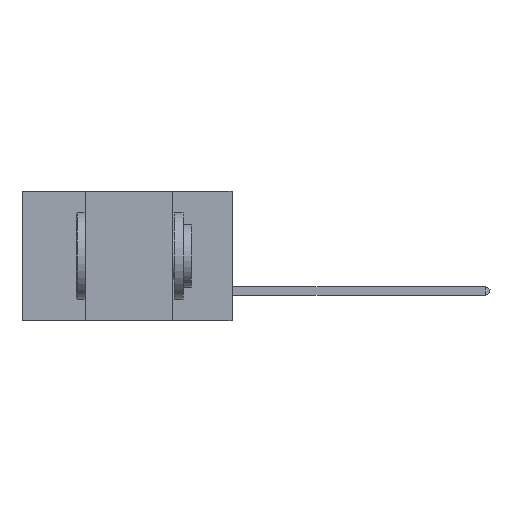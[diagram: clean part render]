
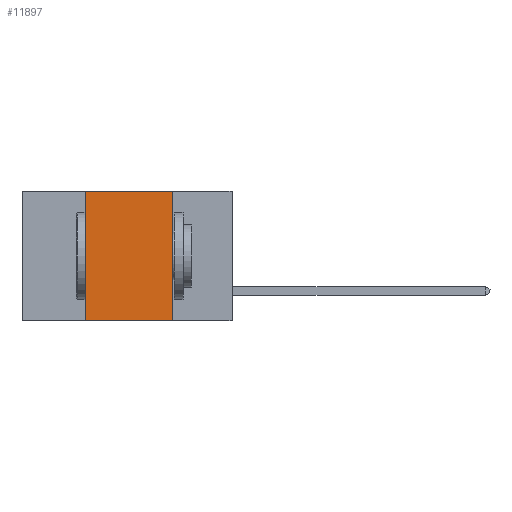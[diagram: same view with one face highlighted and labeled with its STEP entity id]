
A CAD part, left-side view. The second image highlights one B-rep face of the part: STEP entity #11897.
In plain terms, the highlighted planar face has unit normal (-1, 0, 0).
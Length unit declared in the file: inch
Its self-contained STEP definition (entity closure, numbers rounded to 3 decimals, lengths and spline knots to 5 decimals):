
#85 = DIRECTION ( 'NONE',  ( 0., 0., -1. ) ) ;
#560 = LINE ( 'NONE', #10812, #12597 ) ;
#1978 = EDGE_CURVE ( 'NONE', #9811, #10006, #11611, .T. ) ;
#2865 = DIRECTION ( 'NONE',  ( 0., 0., -1. ) ) ;
#2898 = ORIENTED_EDGE ( 'NONE', *, *, #3140, .F. ) ;
#3039 = EDGE_CURVE ( 'NONE', #12158, #3746, #560, .T. ) ;
#3117 = ORIENTED_EDGE ( 'NONE', *, *, #1978, .F. ) ;
#3140 = EDGE_CURVE ( 'NONE', #12158, #9811, #3881, .T. ) ;
#3216 = CARTESIAN_POINT ( 'NONE',  ( 0., 0.6, 0. ) ) ;
#3274 = CARTESIAN_POINT ( 'NONE',  ( 0., 0.17, 0. ) ) ;
#3532 = VECTOR ( 'NONE', #6941, 39.37008 ) ;
#3746 = VERTEX_POINT ( 'NONE', #11236 ) ;
#3881 = LINE ( 'NONE', #4611, #3532 ) ;
#3956 = CARTESIAN_POINT ( 'NONE',  ( 0., 0.42, 0. ) ) ;
#4611 = CARTESIAN_POINT ( 'NONE',  ( 0., 0.42, 0. ) ) ;
#5964 = EDGE_CURVE ( 'NONE', #10006, #3746, #13099, .T. ) ;
#6756 = DIRECTION ( 'NONE',  ( 0., -1., 0. ) ) ;
#6896 = ORIENTED_EDGE ( 'NONE', *, *, #3039, .T. ) ;
#6941 = DIRECTION ( 'NONE',  ( 0., 0., 1. ) ) ;
#7434 = CARTESIAN_POINT ( 'NONE',  ( 0., 0.42, -0.37 ) ) ;
#9105 = PLANE ( 'NONE',  #13553 ) ;
#9153 = CARTESIAN_POINT ( 'NONE',  ( 0., 0.6, 0. ) ) ;
#9622 = ORIENTED_EDGE ( 'NONE', *, *, #5964, .F. ) ;
#9811 = VERTEX_POINT ( 'NONE', #3956 ) ;
#9864 = VECTOR ( 'NONE', #6756, 39.37008 ) ;
#10006 = VERTEX_POINT ( 'NONE', #3274 ) ;
#10125 = VECTOR ( 'NONE', #2865, 39.37008 ) ;
#10812 = CARTESIAN_POINT ( 'NONE',  ( 0., 0.6, -0.37 ) ) ;
#11236 = CARTESIAN_POINT ( 'NONE',  ( 0., 0.17, -0.37 ) ) ;
#11384 = CARTESIAN_POINT ( 'NONE',  ( 0., 0.17, 0. ) ) ;
#11611 = LINE ( 'NONE', #3216, #9864 ) ;
#11897 = ADVANCED_FACE ( 'NONE', ( #11909 ), #9105, .F. ) ;
#11909 = FACE_OUTER_BOUND ( 'NONE', #12701, .T. ) ;
#12158 = VERTEX_POINT ( 'NONE', #7434 ) ;
#12484 = DIRECTION ( 'NONE',  ( 1., 0., 0. ) ) ;
#12597 = VECTOR ( 'NONE', #14159, 39.37008 ) ;
#12701 = EDGE_LOOP ( 'NONE', ( #9622, #3117, #2898, #6896 ) ) ;
#13099 = LINE ( 'NONE', #11384, #10125 ) ;
#13553 = AXIS2_PLACEMENT_3D ( 'NONE', #9153, #12484, #85 ) ;
#14159 = DIRECTION ( 'NONE',  ( 0., -1., 0. ) ) ;
